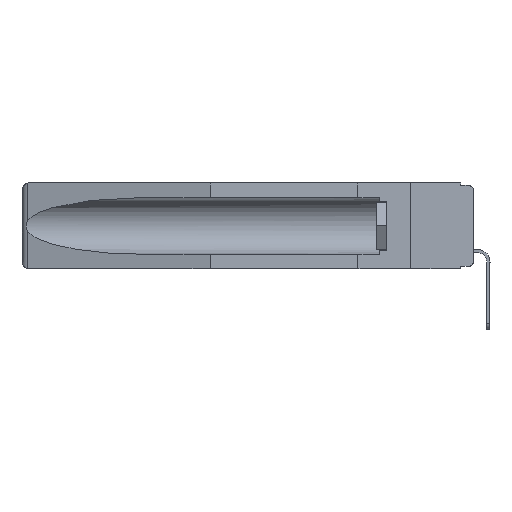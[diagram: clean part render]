
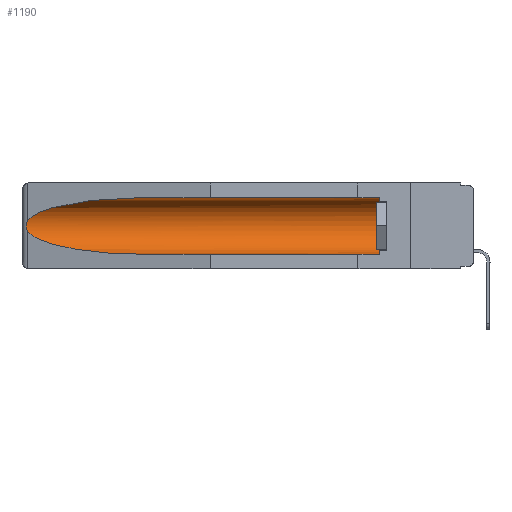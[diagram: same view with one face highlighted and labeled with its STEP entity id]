
A CAD part, left-side view. The second image highlights one B-rep face of the part: STEP entity #1190.
In plain terms, the highlighted cylindrical face has radius 2.857 mm (diameter 5.715 mm), a partial arc.
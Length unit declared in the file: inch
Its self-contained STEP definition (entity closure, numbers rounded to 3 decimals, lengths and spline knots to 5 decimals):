
#442 = CARTESIAN_POINT ( 'NONE',  ( 0.26537, 1.52718, -0.14972 ) ) ;
#522 = CARTESIAN_POINT ( 'NONE',  ( 0.155, 0.126, -0.1715 ) ) ;
#1086 = CARTESIAN_POINT ( 'NONE',  ( 0.155, -0.30754, -0.059 ) ) ;
#1190 = ADVANCED_FACE ( 'NONE', ( #16600 ), #11566, .F. ) ;
#1648 = CARTESIAN_POINT ( 'NONE',  ( 0.2675, 1.53308, -0.16763 ) ) ;
#1819 = AXIS2_PLACEMENT_3D ( 'NONE', #6739, #18247, #10135 ) ;
#2166 = ORIENTED_EDGE ( 'NONE', *, *, #8993, .T. ) ;
#2540 = VERTEX_POINT ( 'NONE', #8203 ) ;
#2638 = ORIENTED_EDGE ( 'NONE', *, *, #20396, .T. ) ;
#2975 = VERTEX_POINT ( 'NONE', #16904 ) ;
#3631 = CARTESIAN_POINT ( 'NONE',  ( 0.26655, 1.53094, -0.18657 ) ) ;
#3937 = DIRECTION ( 'NONE',  ( 0., -1., 0. ) ) ;
#4291 = VERTEX_POINT ( 'NONE', #16715 ) ;
#4412 = VECTOR ( 'NONE', #16357, 39.37008 ) ;
#5146 = CARTESIAN_POINT ( 'NONE',  ( 0.21114, 1.30732, -0.284 ) ) ;
#5166 = CARTESIAN_POINT ( 'NONE',  ( 0.26597, 1.52961, -0.15275 ) ) ;
#5349 = VERTEX_POINT ( 'NONE', #8652 ) ;
#6016 = CARTESIAN_POINT ( 'NONE',  ( 0.26537, 1.52718, -0.14972 ) ) ;
#6169 = ORIENTED_EDGE ( 'NONE', *, *, #10244, .F. ) ;
#6357 = EDGE_LOOP ( 'NONE', ( #19573, #2638, #6602, #6169, #2166, #7469 ) ) ;
#6602 = ORIENTED_EDGE ( 'NONE', *, *, #15190, .T. ) ;
#6613 = CARTESIAN_POINT ( 'NONE',  ( 0.26597, 1.5296, -0.19026 ) ) ;
#6739 = CARTESIAN_POINT ( 'NONE',  ( 0.155, -0.30754, -0.1715 ) ) ;
#7469 = ORIENTED_EDGE ( 'NONE', *, *, #7686, .T. ) ;
#7612 = AXIS2_PLACEMENT_3D ( 'NONE', #522, #3937, #13501 ) ;
#7686 = EDGE_CURVE ( 'NONE', #7918, #2975, #16124, .T. ) ;
#7803 = DIRECTION ( 'NONE',  ( 0., 1., 0. ) ) ;
#7918 = VERTEX_POINT ( 'NONE', #20383 ) ;
#8166 = LINE ( 'NONE', #19759, #4412 ) ;
#8203 = CARTESIAN_POINT ( 'NONE',  ( 0.155, 0.126, -0.284 ) ) ;
#8652 = CARTESIAN_POINT ( 'NONE',  ( 0.26537, 1.52718, -0.19328 ) ) ;
#8702 = CARTESIAN_POINT ( 'NONE',  ( 0.26537, 1.52718, -0.14972 ) ) ;
#8818 = CARTESIAN_POINT ( 'NONE',  ( 0.155, 1.07973, -0.059 ) ) ;
#8993 = EDGE_CURVE ( 'NONE', #2540, #7918, #9371, .T. ) ;
#9371 = CIRCLE ( 'NONE', #7612, 0.1125 ) ;
#10135 = DIRECTION ( 'NONE',  ( 0., 0., 1. ) ) ;
#10243 = CARTESIAN_POINT ( 'NONE',  ( 0.2675, 1.53308, -0.17534 ) ) ;
#10244 = EDGE_CURVE ( 'NONE', #2540, #4291, #8166, .T. ) ;
#10666 = CARTESIAN_POINT ( 'NONE',  ( 0.25451, 1.48313, -0.09465 ) ) ;
#11560 = CARTESIAN_POINT ( 'NONE',  ( 0.2673, 1.5327, -0.16383 ) ) ;
#11566 = CYLINDRICAL_SURFACE ( 'NONE', #1819, 0.1125 ) ;
#12198 =( BOUNDED_CURVE ( )  B_SPLINE_CURVE ( 3, ( #13505, #20175, #5146, #18538 ),
 .UNSPECIFIED., .F., .F. ) 
 B_SPLINE_CURVE_WITH_KNOTS ( ( 4, 4 ),
 ( 0.1948, 1.5708 ),
 .UNSPECIFIED. ) 
 CURVE ( )  GEOMETRIC_REPRESENTATION_ITEM ( )  RATIONAL_B_SPLINE_CURVE ( ( 1., 0.848, 0.848, 1. ) ) 
 REPRESENTATION_ITEM ( '' )  );
#13501 = DIRECTION ( 'NONE',  ( 0., 0., 1. ) ) ;
#13505 = CARTESIAN_POINT ( 'NONE',  ( 0.26537, 1.52718, -0.19328 ) ) ;
#13634 = CARTESIAN_POINT ( 'NONE',  ( 0.26537, 1.52718, -0.19328 ) ) ;
#15190 = EDGE_CURVE ( 'NONE', #5349, #4291, #12198, .T. ) ;
#16124 = LINE ( 'NONE', #1086, #20466 ) ;
#16357 = DIRECTION ( 'NONE',  ( 0., 1., 0. ) ) ;
#16600 = FACE_OUTER_BOUND ( 'NONE', #6357, .T. ) ;
#16697 = CARTESIAN_POINT ( 'NONE',  ( 0.26654, 1.53092, -0.15636 ) ) ;
#16715 = CARTESIAN_POINT ( 'NONE',  ( 0.155, 1.07973, -0.284 ) ) ;
#16904 = CARTESIAN_POINT ( 'NONE',  ( 0.155, 1.07973, -0.059 ) ) ;
#17837 = VERTEX_POINT ( 'NONE', #6016 ) ;
#18247 = DIRECTION ( 'NONE',  ( 0., 1., 0. ) ) ;
#18538 = CARTESIAN_POINT ( 'NONE',  ( 0.155, 1.07973, -0.284 ) ) ;
#18911 =( BOUNDED_CURVE ( )  B_SPLINE_CURVE ( 3, ( #8818, #20416, #10666, #442 ),
 .UNSPECIFIED., .F., .F. ) 
 B_SPLINE_CURVE_WITH_KNOTS ( ( 4, 4 ),
 ( 4.71239, 6.08839 ),
 .UNSPECIFIED. ) 
 CURVE ( )  GEOMETRIC_REPRESENTATION_ITEM ( )  RATIONAL_B_SPLINE_CURVE ( ( 1., 0.848, 0.848, 1. ) ) 
 REPRESENTATION_ITEM ( '' )  );
#19103 = EDGE_CURVE ( 'NONE', #2975, #17837, #18911, .T. ) ;
#19573 = ORIENTED_EDGE ( 'NONE', *, *, #19103, .T. ) ;
#19759 = CARTESIAN_POINT ( 'NONE',  ( 0.155, -0.30754, -0.284 ) ) ;
#20175 = CARTESIAN_POINT ( 'NONE',  ( 0.25451, 1.48313, -0.24835 ) ) ;
#20280 = B_SPLINE_CURVE_WITH_KNOTS ( 'NONE', 3,
 ( #8702, #5166, #16697, #11560, #1648, #10243, #21629, #3631, #6613, #13634 ),
 .UNSPECIFIED., .F., .F.,
 ( 4, 2, 2, 2, 4 ),
 ( 0., 0.00029, 0.00058, 0.00087, 0.00117 ),
 .UNSPECIFIED. ) ;
#20383 = CARTESIAN_POINT ( 'NONE',  ( 0.155, 0.126, -0.059 ) ) ;
#20396 = EDGE_CURVE ( 'NONE', #17837, #5349, #20280, .T. ) ;
#20416 = CARTESIAN_POINT ( 'NONE',  ( 0.21114, 1.30732, -0.059 ) ) ;
#20466 = VECTOR ( 'NONE', #7803, 39.37008 ) ;
#21629 = CARTESIAN_POINT ( 'NONE',  ( 0.2673, 1.53269, -0.17917 ) ) ;
